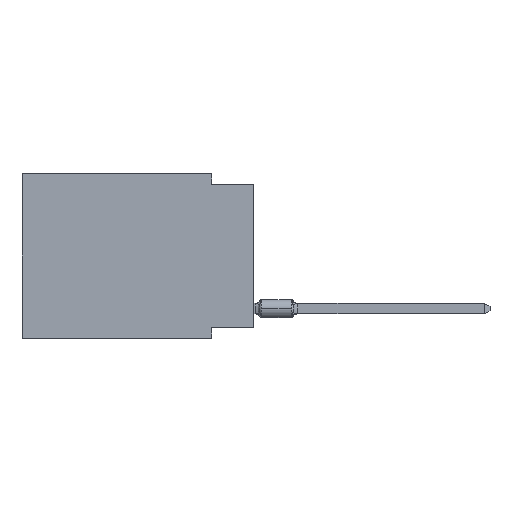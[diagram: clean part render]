
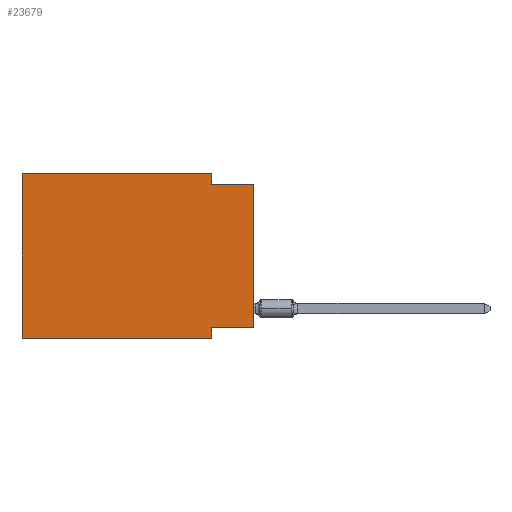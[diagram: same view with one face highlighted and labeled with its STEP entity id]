
A CAD part, left-side view. The second image highlights one B-rep face of the part: STEP entity #23679.
In plain terms, the highlighted planar face has unit normal (-1, 0, 0).
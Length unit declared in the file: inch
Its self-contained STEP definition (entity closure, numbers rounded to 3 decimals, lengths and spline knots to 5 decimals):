
#15 = LINE ( 'NONE', #15666, #10613 ) ;
#583 = VERTEX_POINT ( 'NONE', #6134 ) ;
#772 = EDGE_CURVE ( 'NONE', #8087, #4273, #7604, .T. ) ;
#895 = CARTESIAN_POINT ( 'NONE',  ( 0., 0.55, 0. ) ) ;
#1841 = VECTOR ( 'NONE', #24447, 39.37008 ) ;
#2291 = PLANE ( 'NONE',  #12600 ) ;
#3362 = VECTOR ( 'NONE', #20970, 39.37008 ) ;
#3472 = VECTOR ( 'NONE', #24400, 39.37008 ) ;
#3602 = VECTOR ( 'NONE', #23547, 39.37008 ) ;
#3986 = VECTOR ( 'NONE', #25032, 39.37008 ) ;
#4273 = VERTEX_POINT ( 'NONE', #17982 ) ;
#4967 = ORIENTED_EDGE ( 'NONE', *, *, #13639, .F. ) ;
#5703 = VECTOR ( 'NONE', #12261, 39.37008 ) ;
#5884 = ORIENTED_EDGE ( 'NONE', *, *, #11895, .F. ) ;
#6134 = CARTESIAN_POINT ( 'NONE',  ( 0., 0.55, -0.39 ) ) ;
#6680 = VERTEX_POINT ( 'NONE', #17735 ) ;
#6844 = EDGE_CURVE ( 'NONE', #11453, #8087, #12658, .T. ) ;
#7604 = LINE ( 'NONE', #23379, #3362 ) ;
#8017 = CARTESIAN_POINT ( 'NONE',  ( 0., 0., 0. ) ) ;
#8043 = VECTOR ( 'NONE', #8749, 39.37008 ) ;
#8071 = ORIENTED_EDGE ( 'NONE', *, *, #8931, .F. ) ;
#8087 = VERTEX_POINT ( 'NONE', #18734 ) ;
#8270 = DIRECTION ( 'NONE',  ( 0., 1., 0. ) ) ;
#8436 = CARTESIAN_POINT ( 'NONE',  ( 0., 0.55, 0. ) ) ;
#8749 = DIRECTION ( 'NONE',  ( 0., 0., -1. ) ) ;
#8931 = EDGE_CURVE ( 'NONE', #583, #11453, #12480, .T. ) ;
#9242 = LINE ( 'NONE', #12843, #8043 ) ;
#9776 = CARTESIAN_POINT ( 'NONE',  ( 0., 0., -0.025 ) ) ;
#10613 = VECTOR ( 'NONE', #8270, 39.37008 ) ;
#11201 = CARTESIAN_POINT ( 'NONE',  ( 0., 0.55, 0. ) ) ;
#11453 = VERTEX_POINT ( 'NONE', #11201 ) ;
#11594 = EDGE_CURVE ( 'NONE', #4273, #16802, #24908, .T. ) ;
#11841 = DIRECTION ( 'NONE',  ( 0., 0., -1. ) ) ;
#11895 = EDGE_CURVE ( 'NONE', #22070, #6680, #9242, .T. ) ;
#12261 = DIRECTION ( 'NONE',  ( 0., -1., 0. ) ) ;
#12342 = CARTESIAN_POINT ( 'NONE',  ( 0., 0.55, 0. ) ) ;
#12480 = LINE ( 'NONE', #895, #3472 ) ;
#12600 = AXIS2_PLACEMENT_3D ( 'NONE', #12342, #23778, #11841 ) ;
#12658 = LINE ( 'NONE', #8436, #1841 ) ;
#12843 = CARTESIAN_POINT ( 'NONE',  ( 0., 0.1, -0.39 ) ) ;
#13639 = EDGE_CURVE ( 'NONE', #23198, #22070, #15, .T. ) ;
#14581 = ORIENTED_EDGE ( 'NONE', *, *, #6844, .F. ) ;
#15663 = ORIENTED_EDGE ( 'NONE', *, *, #21147, .T. ) ;
#15666 = CARTESIAN_POINT ( 'NONE',  ( 0., 0., -0.365 ) ) ;
#15741 = CARTESIAN_POINT ( 'NONE',  ( 0., 0., -0.025 ) ) ;
#16044 = CARTESIAN_POINT ( 'NONE',  ( 0., 0.1, -0.365 ) ) ;
#16802 = VERTEX_POINT ( 'NONE', #15741 ) ;
#17735 = CARTESIAN_POINT ( 'NONE',  ( 0., 0.1, -0.39 ) ) ;
#17982 = CARTESIAN_POINT ( 'NONE',  ( 0., 0.1, -0.025 ) ) ;
#18734 = CARTESIAN_POINT ( 'NONE',  ( 0., 0.1, 0. ) ) ;
#18832 = EDGE_LOOP ( 'NONE', ( #15663, #22495, #20376, #14581, #8071, #19172, #5884, #4967 ) ) ;
#19172 = ORIENTED_EDGE ( 'NONE', *, *, #25083, .T. ) ;
#19857 = LINE ( 'NONE', #8017, #3602 ) ;
#20243 = CARTESIAN_POINT ( 'NONE',  ( 0., 0.55, -0.39 ) ) ;
#20376 = ORIENTED_EDGE ( 'NONE', *, *, #772, .F. ) ;
#20970 = DIRECTION ( 'NONE',  ( 0., 0., -1. ) ) ;
#21147 = EDGE_CURVE ( 'NONE', #23198, #16802, #19857, .T. ) ;
#21279 = CARTESIAN_POINT ( 'NONE',  ( 0., 0., -0.365 ) ) ;
#21616 = FACE_OUTER_BOUND ( 'NONE', #18832, .T. ) ;
#22070 = VERTEX_POINT ( 'NONE', #16044 ) ;
#22495 = ORIENTED_EDGE ( 'NONE', *, *, #11594, .F. ) ;
#23198 = VERTEX_POINT ( 'NONE', #21279 ) ;
#23379 = CARTESIAN_POINT ( 'NONE',  ( 0., 0.1, 0. ) ) ;
#23547 = DIRECTION ( 'NONE',  ( 0., 0., 1. ) ) ;
#23679 = ADVANCED_FACE ( 'NONE', ( #21616 ), #2291, .F. ) ;
#23778 = DIRECTION ( 'NONE',  ( 1., 0., 0. ) ) ;
#24051 = LINE ( 'NONE', #20243, #5703 ) ;
#24400 = DIRECTION ( 'NONE',  ( 0., 0., 1. ) ) ;
#24447 = DIRECTION ( 'NONE',  ( 0., -1., 0. ) ) ;
#24908 = LINE ( 'NONE', #9776, #3986 ) ;
#25032 = DIRECTION ( 'NONE',  ( 0., -1., 0. ) ) ;
#25083 = EDGE_CURVE ( 'NONE', #583, #6680, #24051, .T. ) ;
